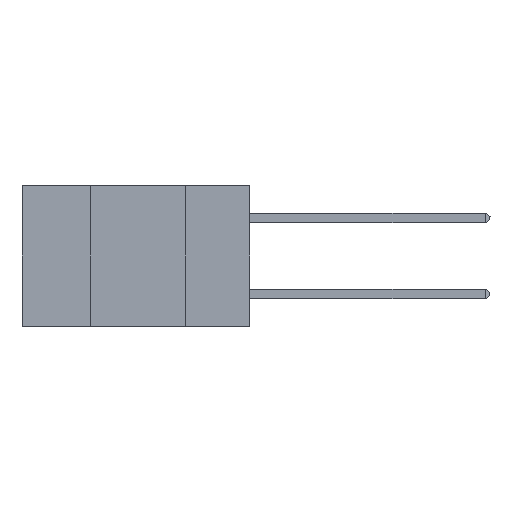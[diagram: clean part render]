
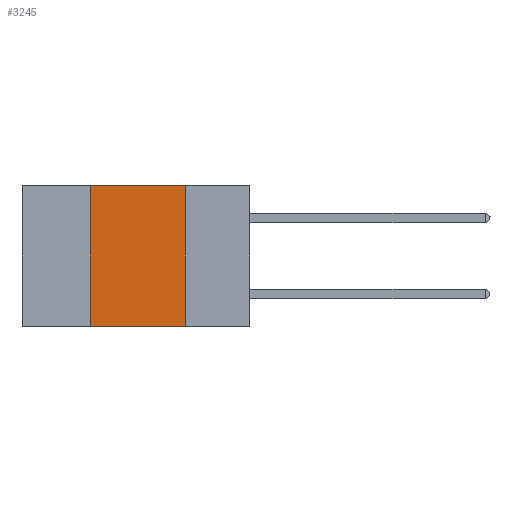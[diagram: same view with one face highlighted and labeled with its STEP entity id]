
A CAD part, left-side view. The second image highlights one B-rep face of the part: STEP entity #3245.
In plain terms, the highlighted planar face has unit normal (-1, 0, 0).
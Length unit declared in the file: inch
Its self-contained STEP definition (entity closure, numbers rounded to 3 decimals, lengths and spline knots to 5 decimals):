
#219 = EDGE_CURVE ( 'NONE', #16779, #922, #3158, .T. ) ;
#327 = ORIENTED_EDGE ( 'NONE', *, *, #219, .F. ) ;
#922 = VERTEX_POINT ( 'NONE', #25093 ) ;
#2405 = ORIENTED_EDGE ( 'NONE', *, *, #11611, .T. ) ;
#3061 = CARTESIAN_POINT ( 'NONE',  ( 0., 0.42, 0. ) ) ;
#3158 = LINE ( 'NONE', #8640, #24032 ) ;
#3245 = ADVANCED_FACE ( 'NONE', ( #11366 ), #20926, .F. ) ;
#3637 = DIRECTION ( 'NONE',  ( 1., 0., 0. ) ) ;
#4064 = DIRECTION ( 'NONE',  ( 0., -1., 0. ) ) ;
#5820 = VERTEX_POINT ( 'NONE', #26103 ) ;
#8640 = CARTESIAN_POINT ( 'NONE',  ( 0., 0.6, 0. ) ) ;
#10278 = DIRECTION ( 'NONE',  ( 0., 0., -1. ) ) ;
#11366 = FACE_OUTER_BOUND ( 'NONE', #15647, .T. ) ;
#11611 = EDGE_CURVE ( 'NONE', #5820, #27139, #27448, .T. ) ;
#11824 = DIRECTION ( 'NONE',  ( 0., 0., -1. ) ) ;
#12548 = EDGE_CURVE ( 'NONE', #922, #27139, #22705, .T. ) ;
#15647 = EDGE_LOOP ( 'NONE', ( #26390, #327, #16002, #2405 ) ) ;
#16002 = ORIENTED_EDGE ( 'NONE', *, *, #27164, .F. ) ;
#16152 = VECTOR ( 'NONE', #4064, 39.37008 ) ;
#16779 = VERTEX_POINT ( 'NONE', #3061 ) ;
#17063 = DIRECTION ( 'NONE',  ( 0., 0., 1. ) ) ;
#17158 = LINE ( 'NONE', #19091, #21132 ) ;
#17437 = AXIS2_PLACEMENT_3D ( 'NONE', #26895, #3637, #10278 ) ;
#18680 = VECTOR ( 'NONE', #11824, 39.37008 ) ;
#18922 = CARTESIAN_POINT ( 'NONE',  ( 0., 0.17, -0.37 ) ) ;
#19091 = CARTESIAN_POINT ( 'NONE',  ( 0., 0.42, 0. ) ) ;
#20926 = PLANE ( 'NONE',  #17437 ) ;
#21132 = VECTOR ( 'NONE', #17063, 39.37008 ) ;
#21437 = DIRECTION ( 'NONE',  ( 0., -1., 0. ) ) ;
#22705 = LINE ( 'NONE', #24547, #18680 ) ;
#23417 = CARTESIAN_POINT ( 'NONE',  ( 0., 0.6, -0.37 ) ) ;
#24032 = VECTOR ( 'NONE', #21437, 39.37008 ) ;
#24547 = CARTESIAN_POINT ( 'NONE',  ( 0., 0.17, 0. ) ) ;
#25093 = CARTESIAN_POINT ( 'NONE',  ( 0., 0.17, 0. ) ) ;
#26103 = CARTESIAN_POINT ( 'NONE',  ( 0., 0.42, -0.37 ) ) ;
#26390 = ORIENTED_EDGE ( 'NONE', *, *, #12548, .F. ) ;
#26895 = CARTESIAN_POINT ( 'NONE',  ( 0., 0.6, 0. ) ) ;
#27139 = VERTEX_POINT ( 'NONE', #18922 ) ;
#27164 = EDGE_CURVE ( 'NONE', #5820, #16779, #17158, .T. ) ;
#27448 = LINE ( 'NONE', #23417, #16152 ) ;
